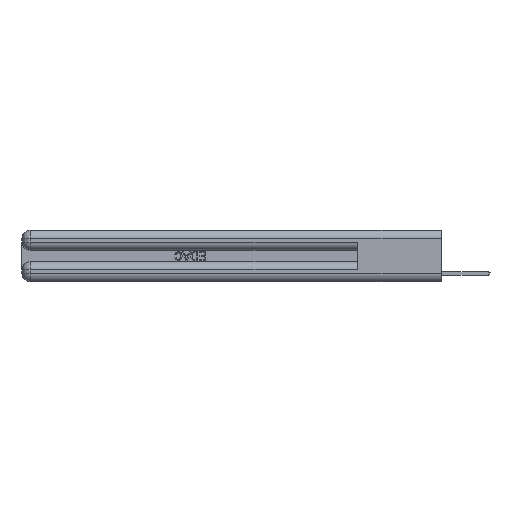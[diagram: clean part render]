
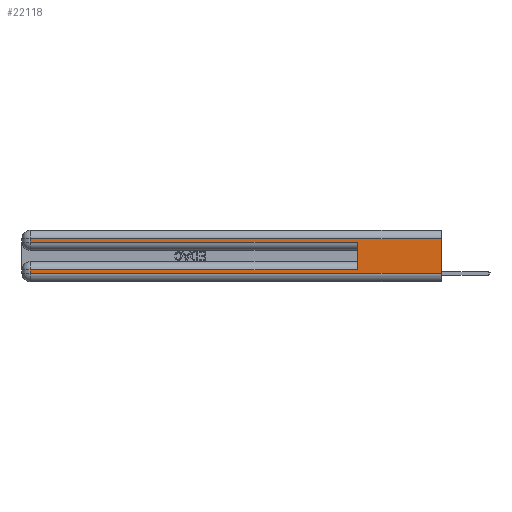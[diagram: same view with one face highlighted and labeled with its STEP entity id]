
A CAD part, left-side view. The second image highlights one B-rep face of the part: STEP entity #22118.
In plain terms, the highlighted planar face has unit normal (-1, 0, 0).
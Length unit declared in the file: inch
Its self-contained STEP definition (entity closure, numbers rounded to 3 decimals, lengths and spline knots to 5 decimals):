
#576 = DIRECTION ( 'NONE',  ( 0., -1., 0. ) ) ;
#821 = CARTESIAN_POINT ( 'NONE',  ( 0., 0.6, 0.145 ) ) ;
#824 = CARTESIAN_POINT ( 'NONE',  ( 0., 0.6, 0.285 ) ) ;
#1055 = EDGE_CURVE ( 'NONE', #16711, #18189, #3795, .T. ) ;
#1599 = ORIENTED_EDGE ( 'NONE', *, *, #25369, .T. ) ;
#2112 = ORIENTED_EDGE ( 'NONE', *, *, #25745, .T. ) ;
#2198 = CARTESIAN_POINT ( 'NONE',  ( 0., 0., 0.31 ) ) ;
#2684 = CARTESIAN_POINT ( 'NONE',  ( 0., 2.94, 0.285 ) ) ;
#2959 = LINE ( 'NONE', #10401, #23965 ) ;
#3795 = LINE ( 'NONE', #16474, #13736 ) ;
#4136 = DIRECTION ( 'NONE',  ( 0., 0., -1. ) ) ;
#4519 = VERTEX_POINT ( 'NONE', #2684 ) ;
#4586 = EDGE_CURVE ( 'NONE', #17487, #12626, #14756, .T. ) ;
#4646 = AXIS2_PLACEMENT_3D ( 'NONE', #24267, #22295, #4136 ) ;
#4833 = DIRECTION ( 'NONE',  ( 0., -1., 0. ) ) ;
#6026 = DIRECTION ( 'NONE',  ( 0., 0., -1. ) ) ;
#6633 = LINE ( 'NONE', #7023, #11743 ) ;
#6898 = EDGE_CURVE ( 'NONE', #16711, #24591, #22054, .T. ) ;
#6997 = CARTESIAN_POINT ( 'NONE',  ( 0., 0., 0.06 ) ) ;
#7023 = CARTESIAN_POINT ( 'NONE',  ( 0., 0., 0.285 ) ) ;
#7437 = VECTOR ( 'NONE', #18736, 39.37008 ) ;
#7907 = CARTESIAN_POINT ( 'NONE',  ( 0., 2.94, 0.31 ) ) ;
#8755 = CARTESIAN_POINT ( 'NONE',  ( 0., 2.94, 0.06 ) ) ;
#9178 = VERTEX_POINT ( 'NONE', #9804 ) ;
#9597 = CARTESIAN_POINT ( 'NONE',  ( 0., 0., 0.06 ) ) ;
#9804 = CARTESIAN_POINT ( 'NONE',  ( 0., 2.94, 0.085 ) ) ;
#10311 = DIRECTION ( 'NONE',  ( 0., 0., -1. ) ) ;
#10325 = DIRECTION ( 'NONE',  ( 0., 1., 0. ) ) ;
#10401 = CARTESIAN_POINT ( 'NONE',  ( 0., 0., 0.085 ) ) ;
#10595 = VECTOR ( 'NONE', #16850, 39.37008 ) ;
#11743 = VECTOR ( 'NONE', #4833, 39.37008 ) ;
#11899 = VECTOR ( 'NONE', #576, 39.37008 ) ;
#12608 = ORIENTED_EDGE ( 'NONE', *, *, #25282, .T. ) ;
#12626 = VERTEX_POINT ( 'NONE', #824 ) ;
#12836 = VECTOR ( 'NONE', #22993, 39.37008 ) ;
#13648 = PLANE ( 'NONE',  #4646 ) ;
#13736 = VECTOR ( 'NONE', #10311, 39.37008 ) ;
#14452 = LINE ( 'NONE', #16277, #16358 ) ;
#14756 = LINE ( 'NONE', #821, #12836 ) ;
#15245 = EDGE_LOOP ( 'NONE', ( #17376, #24639, #2112, #23427, #21518, #12608, #16097, #1599 ) ) ;
#15780 = LINE ( 'NONE', #24316, #7437 ) ;
#16097 = ORIENTED_EDGE ( 'NONE', *, *, #24631, .T. ) ;
#16277 = CARTESIAN_POINT ( 'NONE',  ( 0., 2.94, 0.37 ) ) ;
#16358 = VECTOR ( 'NONE', #6026, 39.37008 ) ;
#16474 = CARTESIAN_POINT ( 'NONE',  ( 0., 0., 0.37 ) ) ;
#16711 = VERTEX_POINT ( 'NONE', #2198 ) ;
#16850 = DIRECTION ( 'NONE',  ( 0., 1., 0. ) ) ;
#17326 = LINE ( 'NONE', #6997, #11899 ) ;
#17376 = ORIENTED_EDGE ( 'NONE', *, *, #1055, .F. ) ;
#17487 = VERTEX_POINT ( 'NONE', #26188 ) ;
#18189 = VERTEX_POINT ( 'NONE', #9597 ) ;
#18736 = DIRECTION ( 'NONE',  ( 0., 0., -1. ) ) ;
#21153 = CARTESIAN_POINT ( 'NONE',  ( 0., 0., 0.31 ) ) ;
#21518 = ORIENTED_EDGE ( 'NONE', *, *, #4586, .F. ) ;
#22054 = LINE ( 'NONE', #21153, #10595 ) ;
#22118 = ADVANCED_FACE ( 'NONE', ( #22237 ), #13648, .F. ) ;
#22237 = FACE_OUTER_BOUND ( 'NONE', #15245, .T. ) ;
#22295 = DIRECTION ( 'NONE',  ( 1., 0., 0. ) ) ;
#22436 = EDGE_CURVE ( 'NONE', #4519, #12626, #6633, .T. ) ;
#22993 = DIRECTION ( 'NONE',  ( 0., 0., 1. ) ) ;
#23427 = ORIENTED_EDGE ( 'NONE', *, *, #22436, .T. ) ;
#23965 = VECTOR ( 'NONE', #10325, 39.37008 ) ;
#24267 = CARTESIAN_POINT ( 'NONE',  ( 0., 0., 0.37 ) ) ;
#24316 = CARTESIAN_POINT ( 'NONE',  ( 0., 2.94, 0.37 ) ) ;
#24591 = VERTEX_POINT ( 'NONE', #7907 ) ;
#24631 = EDGE_CURVE ( 'NONE', #9178, #25875, #15780, .T. ) ;
#24639 = ORIENTED_EDGE ( 'NONE', *, *, #6898, .T. ) ;
#25282 = EDGE_CURVE ( 'NONE', #17487, #9178, #2959, .T. ) ;
#25369 = EDGE_CURVE ( 'NONE', #25875, #18189, #17326, .T. ) ;
#25745 = EDGE_CURVE ( 'NONE', #24591, #4519, #14452, .T. ) ;
#25875 = VERTEX_POINT ( 'NONE', #8755 ) ;
#26188 = CARTESIAN_POINT ( 'NONE',  ( 0., 0.6, 0.085 ) ) ;
